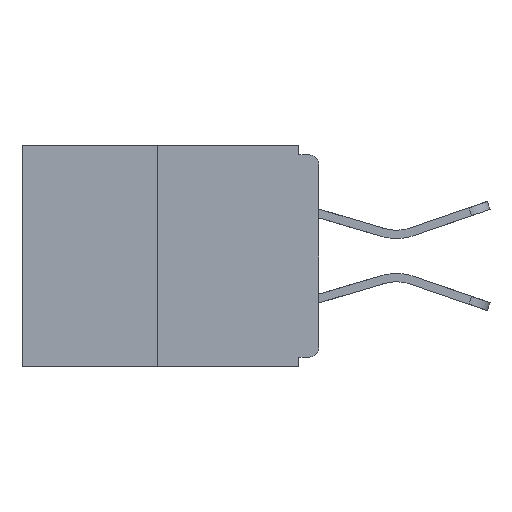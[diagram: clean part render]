
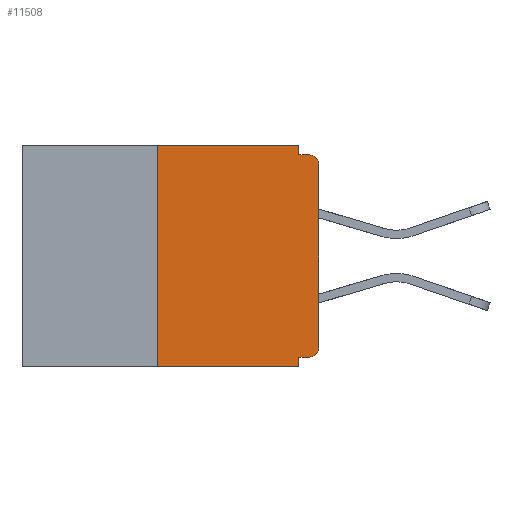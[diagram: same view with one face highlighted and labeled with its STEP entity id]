
A CAD part, left-side view. The second image highlights one B-rep face of the part: STEP entity #11508.
In plain terms, the highlighted planar face has unit normal (-1, 0, 0).
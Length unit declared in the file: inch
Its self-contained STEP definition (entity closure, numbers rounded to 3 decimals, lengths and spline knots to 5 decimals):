
#85 = DIRECTION ( 'NONE',  ( 0., 0., 1. ) ) ;
#113 = VERTEX_POINT ( 'NONE', #8010 ) ;
#218 = CARTESIAN_POINT ( 'NONE',  ( 0., 0.015, -0.313 ) ) ;
#267 = AXIS2_PLACEMENT_3D ( 'NONE', #218, #12418, #18391 ) ;
#617 = EDGE_CURVE ( 'NONE', #3048, #13774, #5405, .T. ) ;
#846 = DIRECTION ( 'NONE',  ( 0., -1., 0. ) ) ;
#850 = ORIENTED_EDGE ( 'NONE', *, *, #3750, .F. ) ;
#982 = VERTEX_POINT ( 'NONE', #4890 ) ;
#1024 = EDGE_CURVE ( 'NONE', #15465, #982, #16014, .T. ) ;
#1508 = VECTOR ( 'NONE', #11447, 39.37008 ) ;
#1575 = VERTEX_POINT ( 'NONE', #10449 ) ;
#1692 = ORIENTED_EDGE ( 'NONE', *, *, #9887, .F. ) ;
#1761 = EDGE_CURVE ( 'NONE', #16742, #13774, #14892, .T. ) ;
#1866 = ORIENTED_EDGE ( 'NONE', *, *, #617, .F. ) ;
#1907 = CARTESIAN_POINT ( 'NONE',  ( 0., 0., -0.313 ) ) ;
#2304 = VECTOR ( 'NONE', #4281, 39.37008 ) ;
#2361 = ORIENTED_EDGE ( 'NONE', *, *, #12239, .T. ) ;
#2576 = VECTOR ( 'NONE', #8803, 39.37008 ) ;
#2775 = CARTESIAN_POINT ( 'NONE',  ( 0., 0.031, -0.343 ) ) ;
#3048 = VERTEX_POINT ( 'NONE', #15502 ) ;
#3218 = LINE ( 'NONE', #9240, #5658 ) ;
#3399 = CIRCLE ( 'NONE', #267, 0.015 ) ;
#3568 = DIRECTION ( 'NONE',  ( -1., 0., 0. ) ) ;
#3750 = EDGE_CURVE ( 'NONE', #5947, #113, #9649, .T. ) ;
#4052 = EDGE_CURVE ( 'NONE', #5947, #4263, #3399, .T. ) ;
#4148 = ORIENTED_EDGE ( 'NONE', *, *, #5581, .F. ) ;
#4263 = VERTEX_POINT ( 'NONE', #1907 ) ;
#4281 = DIRECTION ( 'NONE',  ( 0., -1., 0. ) ) ;
#4641 = ORIENTED_EDGE ( 'NONE', *, *, #1024, .T. ) ;
#4890 = CARTESIAN_POINT ( 'NONE',  ( 0., 0.031, -0.343 ) ) ;
#5405 = LINE ( 'NONE', #16323, #18432 ) ;
#5581 = EDGE_CURVE ( 'NONE', #18592, #1575, #18085, .T. ) ;
#5639 = EDGE_LOOP ( 'NONE', ( #4148, #1692, #4641, #7312, #850, #14117, #2361, #7714, #1866, #6558 ) ) ;
#5658 = VECTOR ( 'NONE', #15315, 39.37008 ) ;
#5760 = DIRECTION ( 'NONE',  ( 0., 0., -1. ) ) ;
#5927 = EDGE_CURVE ( 'NONE', #113, #982, #19548, .T. ) ;
#5947 = VERTEX_POINT ( 'NONE', #10516 ) ;
#6060 = CARTESIAN_POINT ( 'NONE',  ( 0., 0.46, 0. ) ) ;
#6215 = CARTESIAN_POINT ( 'NONE',  ( 0., 0.25, 0. ) ) ;
#6303 = VECTOR ( 'NONE', #85, 39.37008 ) ;
#6367 = CARTESIAN_POINT ( 'NONE',  ( 0., 0.25, -0.343 ) ) ;
#6477 = CARTESIAN_POINT ( 'NONE',  ( 0., 0., -0.03 ) ) ;
#6558 = ORIENTED_EDGE ( 'NONE', *, *, #14501, .F. ) ;
#6940 = DIRECTION ( 'NONE',  ( 0., 0., -1. ) ) ;
#7312 = ORIENTED_EDGE ( 'NONE', *, *, #5927, .F. ) ;
#7714 = ORIENTED_EDGE ( 'NONE', *, *, #1761, .T. ) ;
#8010 = CARTESIAN_POINT ( 'NONE',  ( 0., 0.031, -0.328 ) ) ;
#8224 = FACE_OUTER_BOUND ( 'NONE', #5639, .T. ) ;
#8803 = DIRECTION ( 'NONE',  ( 0., 0., -1. ) ) ;
#8887 = LINE ( 'NONE', #6215, #6303 ) ;
#9240 = CARTESIAN_POINT ( 'NONE',  ( 0., 0., 0. ) ) ;
#9649 = LINE ( 'NONE', #18703, #1508 ) ;
#9887 = EDGE_CURVE ( 'NONE', #15465, #18592, #8887, .T. ) ;
#10008 = CARTESIAN_POINT ( 'NONE',  ( 0., 0.015, -0.015 ) ) ;
#10449 = CARTESIAN_POINT ( 'NONE',  ( 0., 0.031, 0. ) ) ;
#10513 = CARTESIAN_POINT ( 'NONE',  ( 0., 0.25, 0. ) ) ;
#10516 = CARTESIAN_POINT ( 'NONE',  ( 0., 0.015, -0.328 ) ) ;
#11100 = CARTESIAN_POINT ( 'NONE',  ( 0., 0.015, -0.03 ) ) ;
#11313 = PLANE ( 'NONE',  #12613 ) ;
#11447 = DIRECTION ( 'NONE',  ( 0., 1., 0. ) ) ;
#11508 = ADVANCED_FACE ( 'NONE', ( #8224 ), #11313, .F. ) ;
#12239 = EDGE_CURVE ( 'NONE', #4263, #16742, #3218, .T. ) ;
#12350 = AXIS2_PLACEMENT_3D ( 'NONE', #11100, #3568, #15672 ) ;
#12418 = DIRECTION ( 'NONE',  ( -1., 0., 0. ) ) ;
#12613 = AXIS2_PLACEMENT_3D ( 'NONE', #15990, #12895, #6940 ) ;
#12636 = VECTOR ( 'NONE', #15816, 39.37008 ) ;
#12830 = CARTESIAN_POINT ( 'NONE',  ( 0., 0.46, -0.343 ) ) ;
#12895 = DIRECTION ( 'NONE',  ( 1., 0., 0. ) ) ;
#13302 = LINE ( 'NONE', #19361, #16287 ) ;
#13774 = VERTEX_POINT ( 'NONE', #10008 ) ;
#14117 = ORIENTED_EDGE ( 'NONE', *, *, #4052, .T. ) ;
#14501 = EDGE_CURVE ( 'NONE', #1575, #3048, #13302, .T. ) ;
#14892 = CIRCLE ( 'NONE', #12350, 0.015 ) ;
#15315 = DIRECTION ( 'NONE',  ( 0., 0., 1. ) ) ;
#15465 = VERTEX_POINT ( 'NONE', #6367 ) ;
#15502 = CARTESIAN_POINT ( 'NONE',  ( 0., 0.031, -0.015 ) ) ;
#15672 = DIRECTION ( 'NONE',  ( 0., 0., -1. ) ) ;
#15816 = DIRECTION ( 'NONE',  ( 0., -1., 0. ) ) ;
#15990 = CARTESIAN_POINT ( 'NONE',  ( 0., 0.46, 0. ) ) ;
#16014 = LINE ( 'NONE', #12830, #12636 ) ;
#16287 = VECTOR ( 'NONE', #5760, 39.37008 ) ;
#16323 = CARTESIAN_POINT ( 'NONE',  ( 0., 0., -0.015 ) ) ;
#16742 = VERTEX_POINT ( 'NONE', #6477 ) ;
#18085 = LINE ( 'NONE', #6060, #2304 ) ;
#18391 = DIRECTION ( 'NONE',  ( 0., 0., -1. ) ) ;
#18432 = VECTOR ( 'NONE', #846, 39.37008 ) ;
#18592 = VERTEX_POINT ( 'NONE', #10513 ) ;
#18703 = CARTESIAN_POINT ( 'NONE',  ( 0., 0., -0.328 ) ) ;
#19361 = CARTESIAN_POINT ( 'NONE',  ( 0., 0.031, 0. ) ) ;
#19548 = LINE ( 'NONE', #2775, #2576 ) ;
